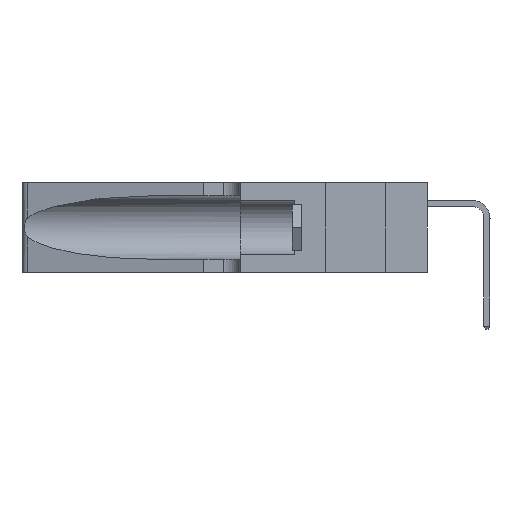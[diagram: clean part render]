
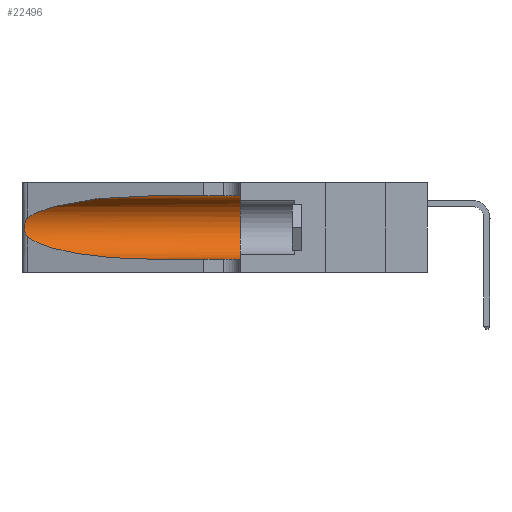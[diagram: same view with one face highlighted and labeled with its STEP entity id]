
A CAD part, left-side view. The second image highlights one B-rep face of the part: STEP entity #22496.
In plain terms, the highlighted cylindrical face has radius 3.308 mm (diameter 6.617 mm), a partial arc.
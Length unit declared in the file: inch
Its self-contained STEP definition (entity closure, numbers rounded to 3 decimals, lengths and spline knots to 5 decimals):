
#511 = ORIENTED_EDGE ( 'NONE', *, *, #15832, .T. ) ;
#694 = ORIENTED_EDGE ( 'NONE', *, *, #9936, .T. ) ;
#900 =( BOUNDED_CURVE ( )  B_SPLINE_CURVE ( 3, ( #13596, #15975, #1977, #18295 ),
 .UNSPECIFIED., .F., .F. ) 
 B_SPLINE_CURVE_WITH_KNOTS ( ( 4, 4 ),
 ( 3.44316, 4.71239 ),
 .UNSPECIFIED. ) 
 CURVE ( )  GEOMETRIC_REPRESENTATION_ITEM ( )  RATIONAL_B_SPLINE_CURVE ( ( 1., 0.87, 0.87, 1. ) ) 
 REPRESENTATION_ITEM ( '' )  );
#1296 = CARTESIAN_POINT ( 'NONE',  ( 0.25555, 1.22994, 0.2215 ) ) ;
#1396 = CARTESIAN_POINT ( 'NONE',  ( 0.25487, 1.22718, 0.14631 ) ) ;
#1531 = CIRCLE ( 'NONE', #18410, 0.13025 ) ;
#1977 = CARTESIAN_POINT ( 'NONE',  ( 0.18966, 0.96281, 0.05475 ) ) ;
#2611 = VERTEX_POINT ( 'NONE', #24754 ) ;
#2790 = ORIENTED_EDGE ( 'NONE', *, *, #27403, .F. ) ;
#3200 = DIRECTION ( 'NONE',  ( 0., 0., -1. ) ) ;
#3541 = B_SPLINE_CURVE_WITH_KNOTS ( 'NONE', 3,
 ( #29271, #1296, #3646, #19951, #5989, #22319, #8343, #24712, #10703, #27050, #13028, #29373, #15381, #1396 ),
 .UNSPECIFIED., .F., .F.,
 ( 4, 2, 2, 2, 2, 2, 4 ),
 ( 0., 0.00027, 0.00053, 0.00107, 0.0016, 0.00187, 0.00214 ),
 .UNSPECIFIED. ) ;
#3646 = CARTESIAN_POINT ( 'NONE',  ( 0.25639, 1.23184, 0.21858 ) ) ;
#5989 = CARTESIAN_POINT ( 'NONE',  ( 0.25854, 1.2359, 0.20912 ) ) ;
#6546 = CARTESIAN_POINT ( 'NONE',  ( 0.1305, 1.61858, 0.05475 ) ) ;
#6608 = LINE ( 'NONE', #9280, #18289 ) ;
#6989 = CARTESIAN_POINT ( 'NONE',  ( 0.25487, 1.22718, 0.22369 ) ) ;
#7788 = ORIENTED_EDGE ( 'NONE', *, *, #24735, .T. ) ;
#7808 = CARTESIAN_POINT ( 'NONE',  ( 0.25487, 1.22718, 0.22369 ) ) ;
#8343 = CARTESIAN_POINT ( 'NONE',  ( 0.26075, 1.23896, 0.19203 ) ) ;
#9030 = CARTESIAN_POINT ( 'NONE',  ( 0.1305, 0.35, 0.31525 ) ) ;
#9280 = CARTESIAN_POINT ( 'NONE',  ( 0.1305, 1.61858, 0.31525 ) ) ;
#9876 = VERTEX_POINT ( 'NONE', #9030 ) ;
#9936 = EDGE_CURVE ( 'NONE', #15140, #24402, #27973, .T. ) ;
#10141 = DIRECTION ( 'NONE',  ( 0., -1., 0. ) ) ;
#10703 = CARTESIAN_POINT ( 'NONE',  ( 0.26017, 1.23833, 0.17102 ) ) ;
#12006 = DIRECTION ( 'NONE',  ( 0., 1., 0. ) ) ;
#12751 = CARTESIAN_POINT ( 'NONE',  ( 0.1305, 0.72297, 0.31525 ) ) ;
#12893 = CARTESIAN_POINT ( 'NONE',  ( 0.25487, 1.22718, 0.14631 ) ) ;
#13028 = CARTESIAN_POINT ( 'NONE',  ( 0.25789, 1.23486, 0.15765 ) ) ;
#13315 = EDGE_CURVE ( 'NONE', #2611, #29424, #17978, .T. ) ;
#13596 = CARTESIAN_POINT ( 'NONE',  ( 0.25487, 1.22718, 0.14631 ) ) ;
#13945 = EDGE_CURVE ( 'NONE', #15140, #9876, #6608, .T. ) ;
#14607 = AXIS2_PLACEMENT_3D ( 'NONE', #17188, #10141, #3200 ) ;
#15140 = VERTEX_POINT ( 'NONE', #12751 ) ;
#15381 = CARTESIAN_POINT ( 'NONE',  ( 0.25555, 1.22993, 0.14849 ) ) ;
#15832 = EDGE_CURVE ( 'NONE', #24402, #26468, #3541, .T. ) ;
#15975 = CARTESIAN_POINT ( 'NONE',  ( 0.2373, 1.15595, 0.08982 ) ) ;
#16081 = FACE_OUTER_BOUND ( 'NONE', #20747, .T. ) ;
#16238 = DIRECTION ( 'NONE',  ( 0., -1., 0. ) ) ;
#17188 = CARTESIAN_POINT ( 'NONE',  ( 0.1305, 1.61858, 0.185 ) ) ;
#17263 = VECTOR ( 'NONE', #25264, 39.37008 ) ;
#17978 = LINE ( 'NONE', #6546, #17263 ) ;
#18289 = VECTOR ( 'NONE', #16238, 39.37008 ) ;
#18295 = CARTESIAN_POINT ( 'NONE',  ( 0.1305, 0.72297, 0.05475 ) ) ;
#18410 = AXIS2_PLACEMENT_3D ( 'NONE', #26032, #12006, #28361 ) ;
#18621 = CARTESIAN_POINT ( 'NONE',  ( 0.2373, 1.15595, 0.28018 ) ) ;
#19747 = CARTESIAN_POINT ( 'NONE',  ( 0.1305, 0.35, 0.05475 ) ) ;
#19951 = CARTESIAN_POINT ( 'NONE',  ( 0.25787, 1.23484, 0.2124 ) ) ;
#20084 = ORIENTED_EDGE ( 'NONE', *, *, #13945, .F. ) ;
#20747 = EDGE_LOOP ( 'NONE', ( #694, #511, #7788, #28156, #2790, #20084 ) ) ;
#20954 = CARTESIAN_POINT ( 'NONE',  ( 0.1305, 0.72297, 0.31525 ) ) ;
#22319 = CARTESIAN_POINT ( 'NONE',  ( 0.26018, 1.23835, 0.19895 ) ) ;
#22496 = ADVANCED_FACE ( 'NONE', ( #16081 ), #26320, .F. ) ;
#24402 = VERTEX_POINT ( 'NONE', #7808 ) ;
#24712 = CARTESIAN_POINT ( 'NONE',  ( 0.26075, 1.23896, 0.178 ) ) ;
#24735 = EDGE_CURVE ( 'NONE', #26468, #2611, #900, .T. ) ;
#24754 = CARTESIAN_POINT ( 'NONE',  ( 0.1305, 0.72297, 0.05475 ) ) ;
#25264 = DIRECTION ( 'NONE',  ( 0., -1., 0. ) ) ;
#26032 = CARTESIAN_POINT ( 'NONE',  ( 0.1305, 0.35, 0.185 ) ) ;
#26320 = CYLINDRICAL_SURFACE ( 'NONE', #14607, 0.13025 ) ;
#26468 = VERTEX_POINT ( 'NONE', #12893 ) ;
#27050 = CARTESIAN_POINT ( 'NONE',  ( 0.25856, 1.23593, 0.16098 ) ) ;
#27403 = EDGE_CURVE ( 'NONE', #9876, #29424, #1531, .T. ) ;
#27937 = CARTESIAN_POINT ( 'NONE',  ( 0.18966, 0.96281, 0.31525 ) ) ;
#27973 =( BOUNDED_CURVE ( )  B_SPLINE_CURVE ( 3, ( #20954, #27937, #18621, #6989 ),
 .UNSPECIFIED., .F., .F. ) 
 B_SPLINE_CURVE_WITH_KNOTS ( ( 4, 4 ),
 ( 1.5708, 2.84003 ),
 .UNSPECIFIED. ) 
 CURVE ( )  GEOMETRIC_REPRESENTATION_ITEM ( )  RATIONAL_B_SPLINE_CURVE ( ( 1., 0.87, 0.87, 1. ) ) 
 REPRESENTATION_ITEM ( '' )  );
#28156 = ORIENTED_EDGE ( 'NONE', *, *, #13315, .T. ) ;
#28361 = DIRECTION ( 'NONE',  ( 0., 0., 1. ) ) ;
#29271 = CARTESIAN_POINT ( 'NONE',  ( 0.25487, 1.22718, 0.22369 ) ) ;
#29373 = CARTESIAN_POINT ( 'NONE',  ( 0.25639, 1.23186, 0.15144 ) ) ;
#29424 = VERTEX_POINT ( 'NONE', #19747 ) ;
